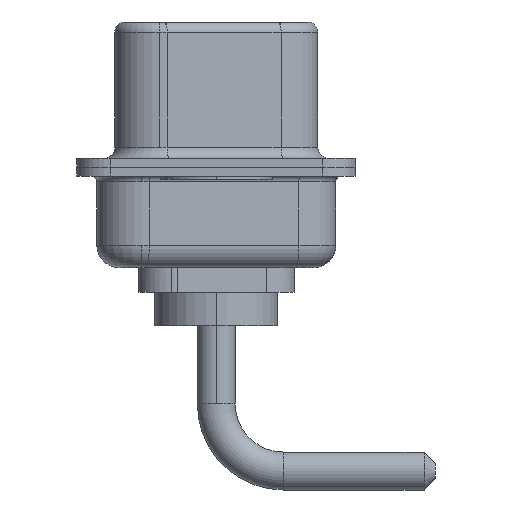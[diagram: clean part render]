
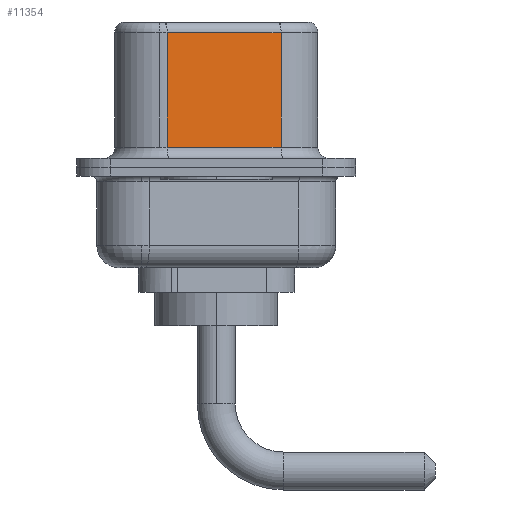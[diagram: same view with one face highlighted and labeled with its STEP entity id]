
A CAD part, left-side view. The second image highlights one B-rep face of the part: STEP entity #11354.
In plain terms, the highlighted planar face has unit normal (-0.985, -0.174, 0).
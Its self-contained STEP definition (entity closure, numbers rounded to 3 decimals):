
#18 = LINE ( 'NONE', #4431, #2375 ) ;
#272 = CARTESIAN_POINT ( 'NONE',  ( 4.58, -2.897, 6.02 ) ) ;
#1195 = DIRECTION ( 'NONE',  ( 0., 0., -1. ) ) ;
#1278 = LINE ( 'NONE', #12118, #13279 ) ;
#2221 = DIRECTION ( 'NONE',  ( 0., 0., -1. ) ) ;
#2295 = EDGE_CURVE ( 'NONE', #7532, #10161, #1278, .T. ) ;
#2375 = VECTOR ( 'NONE', #4641, 1000. ) ;
#3043 = EDGE_LOOP ( 'NONE', ( #4895, #7580, #13001, #10715 ) ) ;
#3131 = DIRECTION ( 'NONE',  ( -0.174, 0.985, 0. ) ) ;
#4271 = CARTESIAN_POINT ( 'NONE',  ( 3.68, 2.203, 0.9 ) ) ;
#4431 = CARTESIAN_POINT ( 'NONE',  ( 4.58, -2.897, 6.02 ) ) ;
#4641 = DIRECTION ( 'NONE',  ( -0.174, 0.985, 0. ) ) ;
#4895 = ORIENTED_EDGE ( 'NONE', *, *, #2295, .F. ) ;
#5033 = VERTEX_POINT ( 'NONE', #8753 ) ;
#5392 = DIRECTION ( 'NONE',  ( 0.174, -0.985, 0. ) ) ;
#6165 = DIRECTION ( 'NONE',  ( 0.985, 0.174, 0. ) ) ;
#6482 = AXIS2_PLACEMENT_3D ( 'NONE', #8334, #6165, #3131 ) ;
#6508 = VECTOR ( 'NONE', #5392, 1000. ) ;
#7532 = VERTEX_POINT ( 'NONE', #272 ) ;
#7580 = ORIENTED_EDGE ( 'NONE', *, *, #14152, .T. ) ;
#7756 = LINE ( 'NONE', #11088, #12088 ) ;
#8334 = CARTESIAN_POINT ( 'NONE',  ( 4.58, -2.897, 6.52 ) ) ;
#8556 = VERTEX_POINT ( 'NONE', #4271 ) ;
#8647 = CARTESIAN_POINT ( 'NONE',  ( 4.58, -2.897, 0.9 ) ) ;
#8753 = CARTESIAN_POINT ( 'NONE',  ( 3.68, 2.203, 6.02 ) ) ;
#9417 = FACE_OUTER_BOUND ( 'NONE', #3043, .T. ) ;
#9724 = LINE ( 'NONE', #8647, #6508 ) ;
#10161 = VERTEX_POINT ( 'NONE', #14266 ) ;
#10715 = ORIENTED_EDGE ( 'NONE', *, *, #12847, .T. ) ;
#11088 = CARTESIAN_POINT ( 'NONE',  ( 3.68, 2.203, 6.52 ) ) ;
#11354 = ADVANCED_FACE ( 'NONE', ( #9417 ), #13043, .F. ) ;
#12088 = VECTOR ( 'NONE', #1195, 1000. ) ;
#12118 = CARTESIAN_POINT ( 'NONE',  ( 4.58, -2.897, 6.52 ) ) ;
#12847 = EDGE_CURVE ( 'NONE', #8556, #10161, #9724, .T. ) ;
#13001 = ORIENTED_EDGE ( 'NONE', *, *, #13759, .T. ) ;
#13043 = PLANE ( 'NONE',  #6482 ) ;
#13279 = VECTOR ( 'NONE', #2221, 1000. ) ;
#13759 = EDGE_CURVE ( 'NONE', #5033, #8556, #7756, .T. ) ;
#14152 = EDGE_CURVE ( 'NONE', #7532, #5033, #18, .T. ) ;
#14266 = CARTESIAN_POINT ( 'NONE',  ( 4.58, -2.897, 0.9 ) ) ;
